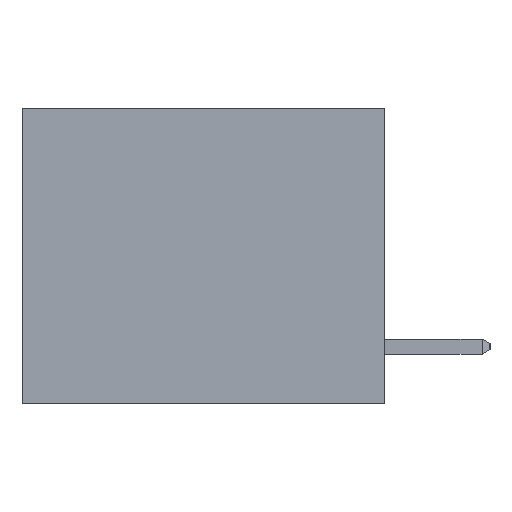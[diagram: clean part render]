
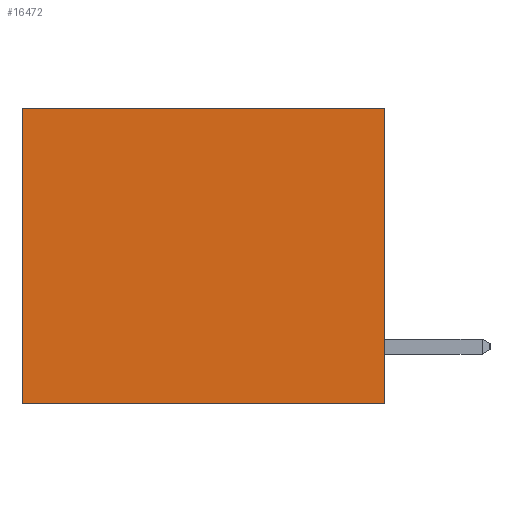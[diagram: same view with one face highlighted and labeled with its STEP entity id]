
A CAD part, left-side view. The second image highlights one B-rep face of the part: STEP entity #16472.
In plain terms, the highlighted planar face has unit normal (-1, 0, 0).
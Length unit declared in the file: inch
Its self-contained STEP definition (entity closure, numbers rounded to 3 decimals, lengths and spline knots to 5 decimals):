
#211 = EDGE_CURVE ( 'NONE', #20504, #21297, #17255, .T. ) ;
#497 = CARTESIAN_POINT ( 'NONE',  ( 0.3165, 0.6, -0.49 ) ) ;
#1553 = CARTESIAN_POINT ( 'NONE',  ( 0.3165, 0., 0. ) ) ;
#1722 = CARTESIAN_POINT ( 'NONE',  ( 0.3165, 0., -0.49 ) ) ;
#2423 = CARTESIAN_POINT ( 'NONE',  ( 0.3165, 0., -0.49 ) ) ;
#4473 = ORIENTED_EDGE ( 'NONE', *, *, #18017, .T. ) ;
#5190 = EDGE_CURVE ( 'NONE', #5337, #12613, #23415, .T. ) ;
#5272 = LINE ( 'NONE', #2423, #25129 ) ;
#5337 = VERTEX_POINT ( 'NONE', #27555 ) ;
#6592 = CARTESIAN_POINT ( 'NONE',  ( 0.3165, 0., 0. ) ) ;
#7164 = VECTOR ( 'NONE', #26030, 39.37008 ) ;
#8398 = ORIENTED_EDGE ( 'NONE', *, *, #211, .T. ) ;
#11582 = DIRECTION ( 'NONE',  ( 0., 0., -1. ) ) ;
#11870 = EDGE_LOOP ( 'NONE', ( #4473, #20713, #23180, #8398 ) ) ;
#11966 = CARTESIAN_POINT ( 'NONE',  ( 0.3165, 0., -0.49 ) ) ;
#12613 = VERTEX_POINT ( 'NONE', #497 ) ;
#13348 = DIRECTION ( 'NONE',  ( 0., 0., -1. ) ) ;
#15579 = EDGE_CURVE ( 'NONE', #20504, #5337, #5272, .T. ) ;
#16472 = ADVANCED_FACE ( 'NONE', ( #16719 ), #27476, .F. ) ;
#16651 = VECTOR ( 'NONE', #11582, 39.37008 ) ;
#16719 = FACE_OUTER_BOUND ( 'NONE', #11870, .T. ) ;
#17255 = LINE ( 'NONE', #6592, #7164 ) ;
#18017 = EDGE_CURVE ( 'NONE', #21297, #12613, #22988, .T. ) ;
#18744 = DIRECTION ( 'NONE',  ( 1., 0., 0. ) ) ;
#18917 = DIRECTION ( 'NONE',  ( 0., 0., -1. ) ) ;
#20504 = VERTEX_POINT ( 'NONE', #1553 ) ;
#20713 = ORIENTED_EDGE ( 'NONE', *, *, #5190, .F. ) ;
#21297 = VERTEX_POINT ( 'NONE', #24907 ) ;
#22281 = AXIS2_PLACEMENT_3D ( 'NONE', #1722, #18744, #18917 ) ;
#22988 = LINE ( 'NONE', #24636, #16651 ) ;
#23180 = ORIENTED_EDGE ( 'NONE', *, *, #15579, .F. ) ;
#23415 = LINE ( 'NONE', #11966, #24769 ) ;
#24636 = CARTESIAN_POINT ( 'NONE',  ( 0.3165, 0.6, -0.49 ) ) ;
#24769 = VECTOR ( 'NONE', #26994, 39.37008 ) ;
#24907 = CARTESIAN_POINT ( 'NONE',  ( 0.3165, 0.6, 0. ) ) ;
#25129 = VECTOR ( 'NONE', #13348, 39.37008 ) ;
#26030 = DIRECTION ( 'NONE',  ( 0., 1., 0. ) ) ;
#26994 = DIRECTION ( 'NONE',  ( 0., 1., 0. ) ) ;
#27476 = PLANE ( 'NONE',  #22281 ) ;
#27555 = CARTESIAN_POINT ( 'NONE',  ( 0.3165, 0., -0.49 ) ) ;
